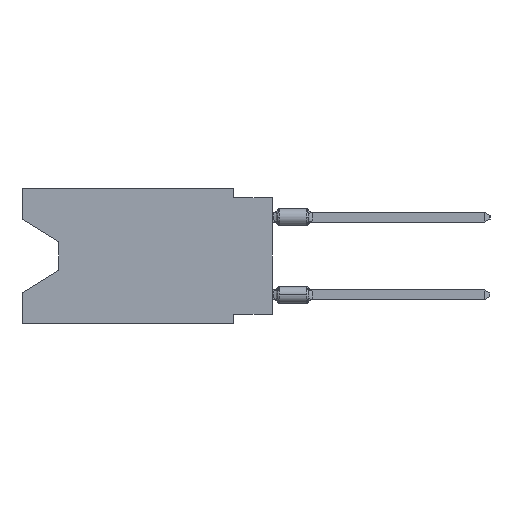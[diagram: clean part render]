
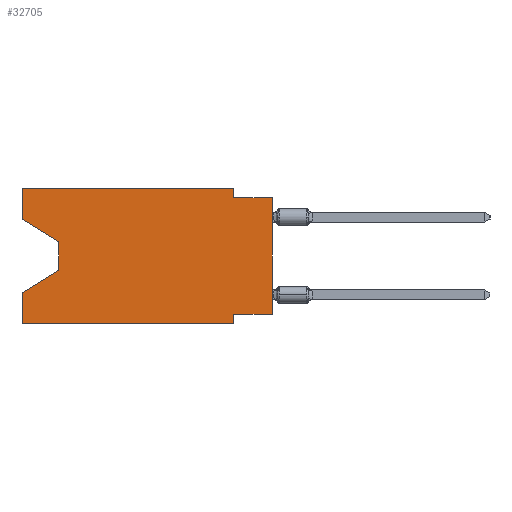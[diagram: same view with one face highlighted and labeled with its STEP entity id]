
A CAD part, left-side view. The second image highlights one B-rep face of the part: STEP entity #32705.
In plain terms, the highlighted planar face has unit normal (-1, 0, 0).
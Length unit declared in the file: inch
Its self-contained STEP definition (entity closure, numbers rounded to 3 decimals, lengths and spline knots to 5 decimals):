
#800 = CARTESIAN_POINT ( 'NONE',  ( 0., 0.55, -0.138 ) ) ;
#2032 = VERTEX_POINT ( 'NONE', #54883 ) ;
#2151 = DIRECTION ( 'NONE',  ( 0., 0.855, -0.519 ) ) ;
#2757 = CARTESIAN_POINT ( 'NONE',  ( 0., 0.1, 0. ) ) ;
#4081 = DIRECTION ( 'NONE',  ( 0., 0., 1. ) ) ;
#4272 = LINE ( 'NONE', #53299, #36434 ) ;
#6174 = DIRECTION ( 'NONE',  ( 0., 0., -1. ) ) ;
#7965 = DIRECTION ( 'NONE',  ( 0., 0., -1. ) ) ;
#8147 = CARTESIAN_POINT ( 'NONE',  ( 0., 0.1, 0. ) ) ;
#8608 = ORIENTED_EDGE ( 'NONE', *, *, #15772, .T. ) ;
#8795 = VECTOR ( 'NONE', #15794, 39.37008 ) ;
#9157 = EDGE_CURVE ( 'NONE', #18463, #47668, #50021, .T. ) ;
#9216 = CARTESIAN_POINT ( 'NONE',  ( 0., 0.645, 0. ) ) ;
#9788 = CARTESIAN_POINT ( 'NONE',  ( 0., 0.645, -0.08025 ) ) ;
#10609 = LINE ( 'NONE', #39397, #30356 ) ;
#10735 = VECTOR ( 'NONE', #43196, 39.37008 ) ;
#12217 = LINE ( 'NONE', #2757, #25282 ) ;
#12714 = ORIENTED_EDGE ( 'NONE', *, *, #55198, .F. ) ;
#13788 = VECTOR ( 'NONE', #55253, 39.37008 ) ;
#13898 = CARTESIAN_POINT ( 'NONE',  ( 0., 0.645, 0. ) ) ;
#15772 = EDGE_CURVE ( 'NONE', #52485, #41593, #4272, .T. ) ;
#15794 = DIRECTION ( 'NONE',  ( 0., 0., -1. ) ) ;
#15913 = CARTESIAN_POINT ( 'NONE',  ( 0., 0.1, -0.325 ) ) ;
#17013 = ORIENTED_EDGE ( 'NONE', *, *, #20746, .F. ) ;
#17408 = CARTESIAN_POINT ( 'NONE',  ( 0., 0., -0.325 ) ) ;
#18225 = DIRECTION ( 'NONE',  ( 0., -1., 0. ) ) ;
#18463 = VERTEX_POINT ( 'NONE', #64481 ) ;
#19193 = VECTOR ( 'NONE', #2151, 39.37008 ) ;
#19517 = LINE ( 'NONE', #29284, #32383 ) ;
#19748 = VERTEX_POINT ( 'NONE', #9788 ) ;
#20746 = EDGE_CURVE ( 'NONE', #51833, #30823, #12217, .T. ) ;
#22787 = VERTEX_POINT ( 'NONE', #22872 ) ;
#22872 = CARTESIAN_POINT ( 'NONE',  ( 0., 0.55, -0.212 ) ) ;
#22981 = ORIENTED_EDGE ( 'NONE', *, *, #9157, .T. ) ;
#24966 = EDGE_CURVE ( 'NONE', #22787, #61319, #26679, .T. ) ;
#25282 = VECTOR ( 'NONE', #7965, 39.37008 ) ;
#25321 = EDGE_CURVE ( 'NONE', #59441, #22787, #25636, .T. ) ;
#25536 = CARTESIAN_POINT ( 'NONE',  ( 0., 0., 0. ) ) ;
#25636 = LINE ( 'NONE', #800, #8795 ) ;
#26125 = ORIENTED_EDGE ( 'NONE', *, *, #24966, .T. ) ;
#26679 = LINE ( 'NONE', #61928, #19193 ) ;
#27006 = ORIENTED_EDGE ( 'NONE', *, *, #39341, .F. ) ;
#28162 = LINE ( 'NONE', #17408, #10735 ) ;
#28239 = VECTOR ( 'NONE', #59773, 39.37008 ) ;
#28741 = ORIENTED_EDGE ( 'NONE', *, *, #40611, .F. ) ;
#29284 = CARTESIAN_POINT ( 'NONE',  ( 0., 0., -0.025 ) ) ;
#29646 = CARTESIAN_POINT ( 'NONE',  ( 0., 0.645, 0. ) ) ;
#30356 = VECTOR ( 'NONE', #55706, 39.37008 ) ;
#30823 = VERTEX_POINT ( 'NONE', #39911 ) ;
#30870 = ORIENTED_EDGE ( 'NONE', *, *, #25321, .T. ) ;
#31356 = VECTOR ( 'NONE', #6174, 39.37008 ) ;
#32383 = VECTOR ( 'NONE', #18225, 39.37008 ) ;
#32705 = ADVANCED_FACE ( 'NONE', ( #49898 ), #44357, .F. ) ;
#32808 = VECTOR ( 'NONE', #35027, 39.37008 ) ;
#35027 = DIRECTION ( 'NONE',  ( 0., 0., 1. ) ) ;
#36265 = AXIS2_PLACEMENT_3D ( 'NONE', #29646, #40414, #45311 ) ;
#36434 = VECTOR ( 'NONE', #58515, 39.37008 ) ;
#39341 = EDGE_CURVE ( 'NONE', #18463, #59226, #28162, .T. ) ;
#39397 = CARTESIAN_POINT ( 'NONE',  ( 0., 0.645, 0. ) ) ;
#39845 = LINE ( 'NONE', #58813, #28239 ) ;
#39863 = ORIENTED_EDGE ( 'NONE', *, *, #48327, .F. ) ;
#39911 = CARTESIAN_POINT ( 'NONE',  ( 0., 0.1, -0.025 ) ) ;
#40414 = DIRECTION ( 'NONE',  ( 1., 0., 0. ) ) ;
#40496 = VECTOR ( 'NONE', #4081, 39.37008 ) ;
#40611 = EDGE_CURVE ( 'NONE', #52485, #61319, #45124, .T. ) ;
#41593 = VERTEX_POINT ( 'NONE', #56319 ) ;
#41687 = LINE ( 'NONE', #13898, #40496 ) ;
#42845 = CARTESIAN_POINT ( 'NONE',  ( 0., 0.645, -0.26975 ) ) ;
#43196 = DIRECTION ( 'NONE',  ( 0., 1., 0. ) ) ;
#44357 = PLANE ( 'NONE',  #36265 ) ;
#44838 = ORIENTED_EDGE ( 'NONE', *, *, #62392, .T. ) ;
#45124 = LINE ( 'NONE', #9216, #32808 ) ;
#45311 = DIRECTION ( 'NONE',  ( 0., 0., -1. ) ) ;
#45568 = ORIENTED_EDGE ( 'NONE', *, *, #49799, .F. ) ;
#46012 = LINE ( 'NONE', #55854, #31356 ) ;
#47668 = VERTEX_POINT ( 'NONE', #55909 ) ;
#48327 = EDGE_CURVE ( 'NONE', #30823, #47668, #19517, .T. ) ;
#49799 = EDGE_CURVE ( 'NONE', #19748, #2032, #41687, .T. ) ;
#49898 = FACE_OUTER_BOUND ( 'NONE', #63369, .T. ) ;
#50021 = LINE ( 'NONE', #25536, #13788 ) ;
#51134 = CARTESIAN_POINT ( 'NONE',  ( 0., 0.645, -0.35 ) ) ;
#51833 = VERTEX_POINT ( 'NONE', #8147 ) ;
#52485 = VERTEX_POINT ( 'NONE', #51134 ) ;
#53299 = CARTESIAN_POINT ( 'NONE',  ( 0., 0.645, -0.35 ) ) ;
#53454 = CARTESIAN_POINT ( 'NONE',  ( 0., 0.55, -0.138 ) ) ;
#54883 = CARTESIAN_POINT ( 'NONE',  ( 0., 0.645, 0. ) ) ;
#55198 = EDGE_CURVE ( 'NONE', #2032, #51833, #10609, .T. ) ;
#55253 = DIRECTION ( 'NONE',  ( 0., 0., 1. ) ) ;
#55706 = DIRECTION ( 'NONE',  ( 0., -1., 0. ) ) ;
#55854 = CARTESIAN_POINT ( 'NONE',  ( 0., 0.1, -0.35 ) ) ;
#55909 = CARTESIAN_POINT ( 'NONE',  ( 0., 0., -0.025 ) ) ;
#56207 = ORIENTED_EDGE ( 'NONE', *, *, #62469, .F. ) ;
#56319 = CARTESIAN_POINT ( 'NONE',  ( 0., 0.1, -0.35 ) ) ;
#58515 = DIRECTION ( 'NONE',  ( 0., -1., 0. ) ) ;
#58813 = CARTESIAN_POINT ( 'NONE',  ( 0., 0.645, -0.08025 ) ) ;
#59226 = VERTEX_POINT ( 'NONE', #15913 ) ;
#59441 = VERTEX_POINT ( 'NONE', #53454 ) ;
#59773 = DIRECTION ( 'NONE',  ( 0., -0.855, -0.519 ) ) ;
#61319 = VERTEX_POINT ( 'NONE', #42845 ) ;
#61928 = CARTESIAN_POINT ( 'NONE',  ( 0., 0.55, -0.212 ) ) ;
#62392 = EDGE_CURVE ( 'NONE', #19748, #59441, #39845, .T. ) ;
#62469 = EDGE_CURVE ( 'NONE', #59226, #41593, #46012, .T. ) ;
#63369 = EDGE_LOOP ( 'NONE', ( #44838, #30870, #26125, #28741, #8608, #56207, #27006, #22981, #39863, #17013, #12714, #45568 ) ) ;
#64481 = CARTESIAN_POINT ( 'NONE',  ( 0., 0., -0.325 ) ) ;
